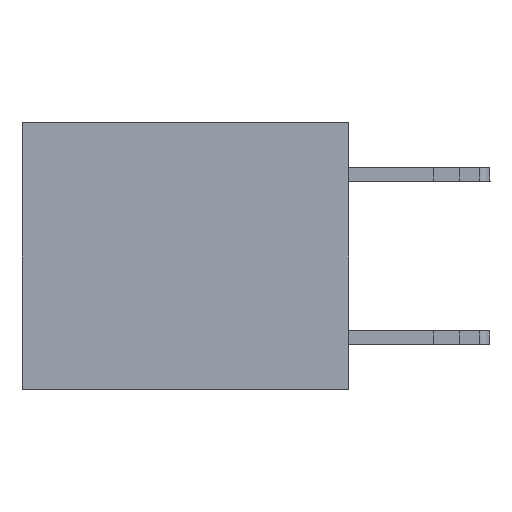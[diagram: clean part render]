
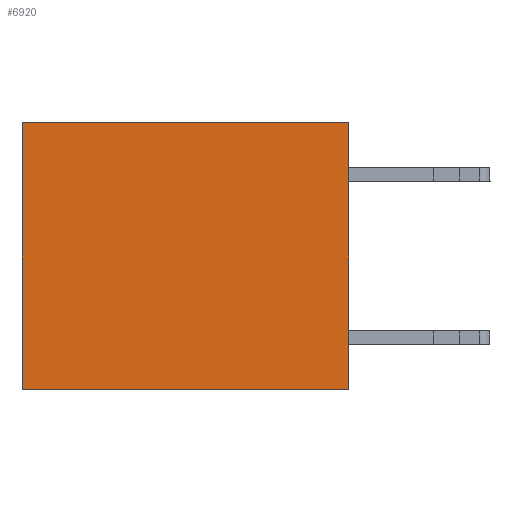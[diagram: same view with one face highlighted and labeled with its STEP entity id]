
A CAD part, left-side view. The second image highlights one B-rep face of the part: STEP entity #6920.
In plain terms, the highlighted planar face has unit normal (-1, 0, 0).
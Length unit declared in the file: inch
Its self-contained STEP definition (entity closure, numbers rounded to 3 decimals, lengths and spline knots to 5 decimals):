
#826 = DIRECTION ( 'NONE',  ( 1., 0., 0. ) ) ;
#3249 = DIRECTION ( 'NONE',  ( 0., 0., -1. ) ) ;
#3730 = VECTOR ( 'NONE', #5563, 39.37008 ) ;
#4935 = CARTESIAN_POINT ( 'NONE',  ( 0.3165, 0., -0.49 ) ) ;
#5069 = AXIS2_PLACEMENT_3D ( 'NONE', #9955, #826, #3249 ) ;
#5192 = CARTESIAN_POINT ( 'NONE',  ( 0.3165, 0.6, -0.49 ) ) ;
#5476 = ORIENTED_EDGE ( 'NONE', *, *, #24199, .T. ) ;
#5563 = DIRECTION ( 'NONE',  ( 0., 1., 0. ) ) ;
#6920 = ADVANCED_FACE ( 'NONE', ( #17049 ), #7578, .F. ) ;
#7332 = ORIENTED_EDGE ( 'NONE', *, *, #8673, .F. ) ;
#7380 = VECTOR ( 'NONE', #14430, 39.37008 ) ;
#7578 = PLANE ( 'NONE',  #5069 ) ;
#8673 = EDGE_CURVE ( 'NONE', #14232, #20117, #9131, .T. ) ;
#9131 = LINE ( 'NONE', #12503, #28612 ) ;
#9493 = CARTESIAN_POINT ( 'NONE',  ( 0.3165, 0.6, -0.49 ) ) ;
#9955 = CARTESIAN_POINT ( 'NONE',  ( 0.3165, 0., -0.49 ) ) ;
#10394 = EDGE_CURVE ( 'NONE', #20117, #29600, #16610, .T. ) ;
#11978 = ORIENTED_EDGE ( 'NONE', *, *, #27629, .T. ) ;
#12382 = CARTESIAN_POINT ( 'NONE',  ( 0.3165, 0., 0. ) ) ;
#12503 = CARTESIAN_POINT ( 'NONE',  ( 0.3165, 0., -0.49 ) ) ;
#13274 = CARTESIAN_POINT ( 'NONE',  ( 0.3165, 0., 0. ) ) ;
#13434 = LINE ( 'NONE', #12382, #3730 ) ;
#14232 = VERTEX_POINT ( 'NONE', #13274 ) ;
#14430 = DIRECTION ( 'NONE',  ( 0., 0., -1. ) ) ;
#14801 = VECTOR ( 'NONE', #23695, 39.37008 ) ;
#15423 = CARTESIAN_POINT ( 'NONE',  ( 0.3165, 0., -0.49 ) ) ;
#16610 = LINE ( 'NONE', #4935, #14801 ) ;
#16886 = VERTEX_POINT ( 'NONE', #28807 ) ;
#17049 = FACE_OUTER_BOUND ( 'NONE', #20771, .T. ) ;
#20117 = VERTEX_POINT ( 'NONE', #15423 ) ;
#20771 = EDGE_LOOP ( 'NONE', ( #5476, #21566, #7332, #11978 ) ) ;
#21566 = ORIENTED_EDGE ( 'NONE', *, *, #10394, .F. ) ;
#23695 = DIRECTION ( 'NONE',  ( 0., 1., 0. ) ) ;
#24199 = EDGE_CURVE ( 'NONE', #16886, #29600, #28644, .T. ) ;
#24253 = DIRECTION ( 'NONE',  ( 0., 0., -1. ) ) ;
#27629 = EDGE_CURVE ( 'NONE', #14232, #16886, #13434, .T. ) ;
#28612 = VECTOR ( 'NONE', #24253, 39.37008 ) ;
#28644 = LINE ( 'NONE', #9493, #7380 ) ;
#28807 = CARTESIAN_POINT ( 'NONE',  ( 0.3165, 0.6, 0. ) ) ;
#29600 = VERTEX_POINT ( 'NONE', #5192 ) ;
